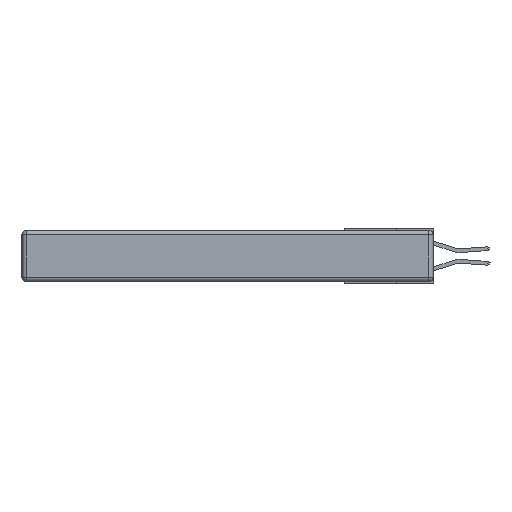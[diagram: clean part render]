
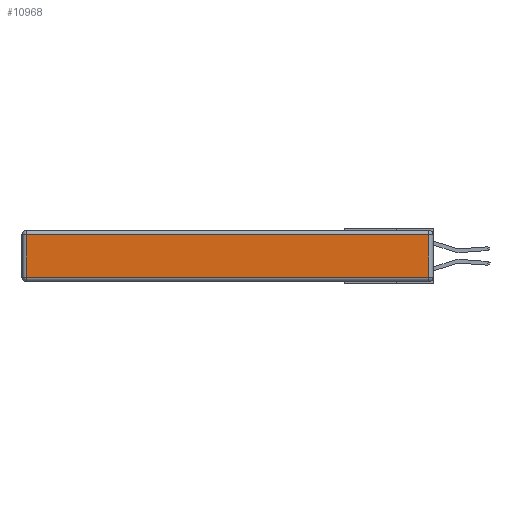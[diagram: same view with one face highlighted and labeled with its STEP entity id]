
A CAD part, left-side view. The second image highlights one B-rep face of the part: STEP entity #10968.
In plain terms, the highlighted planar face has unit normal (-1, 0, 0).
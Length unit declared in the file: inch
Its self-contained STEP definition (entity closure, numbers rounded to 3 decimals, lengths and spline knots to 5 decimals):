
#90 = ORIENTED_EDGE ( 'NONE', *, *, #24380, .T. ) ;
#138 = CARTESIAN_POINT ( 'NONE',  ( 0., 2.72, -0.03 ) ) ;
#202 = ORIENTED_EDGE ( 'NONE', *, *, #21073, .T. ) ;
#293 = DIRECTION ( 'NONE',  ( 0., 0., 1. ) ) ;
#1786 = CARTESIAN_POINT ( 'NONE',  ( 0., 0.03, -0.313 ) ) ;
#2277 = DIRECTION ( 'NONE',  ( 0., 0., 1. ) ) ;
#2505 = EDGE_CURVE ( 'NONE', #21556, #5960, #3916, .T. ) ;
#3487 = EDGE_LOOP ( 'NONE', ( #202, #8925, #90, #23424 ) ) ;
#3916 = LINE ( 'NONE', #18895, #23904 ) ;
#4229 = DIRECTION ( 'NONE',  ( -1., 0., 0. ) ) ;
#5960 = VERTEX_POINT ( 'NONE', #7213 ) ;
#6168 = CARTESIAN_POINT ( 'NONE',  ( 0., 0., -0.343 ) ) ;
#6881 = DIRECTION ( 'NONE',  ( 0., 1., 0. ) ) ;
#6992 = AXIS2_PLACEMENT_3D ( 'NONE', #6168, #4229, #2277 ) ;
#7213 = CARTESIAN_POINT ( 'NONE',  ( 0., 2.72, -0.313 ) ) ;
#8925 = ORIENTED_EDGE ( 'NONE', *, *, #19383, .T. ) ;
#9277 = DIRECTION ( 'NONE',  ( 0., 0., -1. ) ) ;
#10090 = VECTOR ( 'NONE', #16240, 39.37008 ) ;
#10424 = VERTEX_POINT ( 'NONE', #1786 ) ;
#10783 = VERTEX_POINT ( 'NONE', #23175 ) ;
#10968 = ADVANCED_FACE ( 'NONE', ( #22369 ), #14027, .T. ) ;
#11166 = VECTOR ( 'NONE', #6881, 39.37008 ) ;
#14027 = PLANE ( 'NONE',  #6992 ) ;
#15911 = VECTOR ( 'NONE', #293, 39.37008 ) ;
#16240 = DIRECTION ( 'NONE',  ( 0., -1., 0. ) ) ;
#17633 = CARTESIAN_POINT ( 'NONE',  ( 0., 0.03, -0.343 ) ) ;
#18342 = CARTESIAN_POINT ( 'NONE',  ( 0., 0., -0.313 ) ) ;
#18895 = CARTESIAN_POINT ( 'NONE',  ( 0., 2.72, -0.343 ) ) ;
#19383 = EDGE_CURVE ( 'NONE', #10424, #10783, #21674, .T. ) ;
#21073 = EDGE_CURVE ( 'NONE', #5960, #10424, #22209, .T. ) ;
#21556 = VERTEX_POINT ( 'NONE', #138 ) ;
#21674 = LINE ( 'NONE', #17633, #15911 ) ;
#22209 = LINE ( 'NONE', #18342, #10090 ) ;
#22369 = FACE_OUTER_BOUND ( 'NONE', #3487, .T. ) ;
#22557 = CARTESIAN_POINT ( 'NONE',  ( 0., 2.75, -0.03 ) ) ;
#23175 = CARTESIAN_POINT ( 'NONE',  ( 0., 0.03, -0.03 ) ) ;
#23424 = ORIENTED_EDGE ( 'NONE', *, *, #2505, .T. ) ;
#23868 = LINE ( 'NONE', #22557, #11166 ) ;
#23904 = VECTOR ( 'NONE', #9277, 39.37008 ) ;
#24380 = EDGE_CURVE ( 'NONE', #10783, #21556, #23868, .T. ) ;
